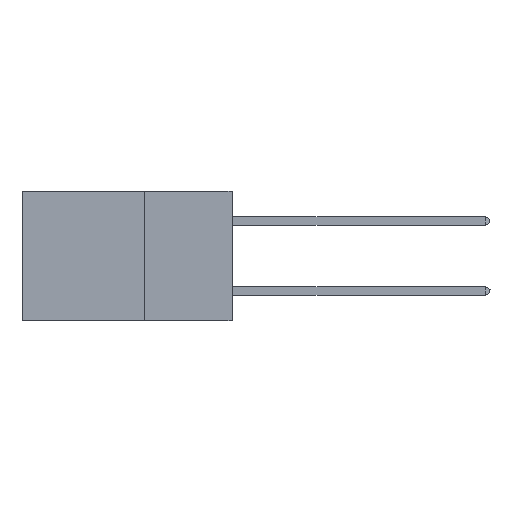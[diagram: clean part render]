
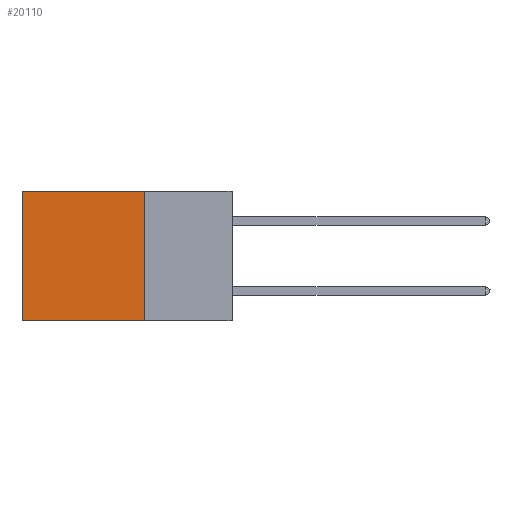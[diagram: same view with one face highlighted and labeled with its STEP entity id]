
A CAD part, left-side view. The second image highlights one B-rep face of the part: STEP entity #20110.
In plain terms, the highlighted planar face has unit normal (-1, 0, 0).
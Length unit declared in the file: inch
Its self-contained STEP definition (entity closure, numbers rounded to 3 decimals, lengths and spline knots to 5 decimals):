
#875 = CARTESIAN_POINT ( 'NONE',  ( 0.2875, 0.25, 0. ) ) ;
#1537 = VECTOR ( 'NONE', #2991, 39.37008 ) ;
#2991 = DIRECTION ( 'NONE',  ( 0., 1., 0. ) ) ;
#4662 = LINE ( 'NONE', #27155, #1537 ) ;
#4837 = EDGE_CURVE ( 'NONE', #18898, #11673, #4662, .T. ) ;
#5326 = LINE ( 'NONE', #6098, #13482 ) ;
#5775 = LINE ( 'NONE', #28295, #11222 ) ;
#5841 = EDGE_CURVE ( 'NONE', #23454, #14903, #29103, .T. ) ;
#6098 = CARTESIAN_POINT ( 'NONE',  ( 0.2875, 0.6, 0. ) ) ;
#6100 = DIRECTION ( 'NONE',  ( 0., 0., -1. ) ) ;
#6164 = EDGE_CURVE ( 'NONE', #11673, #14903, #5326, .T. ) ;
#8176 = DIRECTION ( 'NONE',  ( 1., 0., 0. ) ) ;
#8627 = CARTESIAN_POINT ( 'NONE',  ( 0.2875, 0.6, -0.37 ) ) ;
#9273 = VECTOR ( 'NONE', #24899, 39.37008 ) ;
#11222 = VECTOR ( 'NONE', #17853, 39.37008 ) ;
#11673 = VERTEX_POINT ( 'NONE', #27627 ) ;
#12040 = ORIENTED_EDGE ( 'NONE', *, *, #4837, .T. ) ;
#13482 = VECTOR ( 'NONE', #20738, 39.37008 ) ;
#14249 = ORIENTED_EDGE ( 'NONE', *, *, #6164, .T. ) ;
#14416 = AXIS2_PLACEMENT_3D ( 'NONE', #875, #8176, #6100 ) ;
#14894 = ORIENTED_EDGE ( 'NONE', *, *, #5841, .F. ) ;
#14903 = VERTEX_POINT ( 'NONE', #8627 ) ;
#15842 = CARTESIAN_POINT ( 'NONE',  ( 0.2875, 0.25, 0. ) ) ;
#17853 = DIRECTION ( 'NONE',  ( 0., 0., -1. ) ) ;
#18898 = VERTEX_POINT ( 'NONE', #15842 ) ;
#20110 = ADVANCED_FACE ( 'NONE', ( #25583 ), #28065, .F. ) ;
#20738 = DIRECTION ( 'NONE',  ( 0., 0., -1. ) ) ;
#23401 = EDGE_CURVE ( 'NONE', #18898, #23454, #5775, .T. ) ;
#23454 = VERTEX_POINT ( 'NONE', #28184 ) ;
#23585 = ORIENTED_EDGE ( 'NONE', *, *, #23401, .F. ) ;
#24899 = DIRECTION ( 'NONE',  ( 0., 1., 0. ) ) ;
#25583 = FACE_OUTER_BOUND ( 'NONE', #31408, .T. ) ;
#27155 = CARTESIAN_POINT ( 'NONE',  ( 0.2875, 0.25, 0. ) ) ;
#27627 = CARTESIAN_POINT ( 'NONE',  ( 0.2875, 0.6, 0. ) ) ;
#28065 = PLANE ( 'NONE',  #14416 ) ;
#28184 = CARTESIAN_POINT ( 'NONE',  ( 0.2875, 0.25, -0.37 ) ) ;
#28295 = CARTESIAN_POINT ( 'NONE',  ( 0.2875, 0.25, 0. ) ) ;
#29103 = LINE ( 'NONE', #29704, #9273 ) ;
#29704 = CARTESIAN_POINT ( 'NONE',  ( 0.2875, 0.25, -0.37 ) ) ;
#31408 = EDGE_LOOP ( 'NONE', ( #14249, #14894, #23585, #12040 ) ) ;
